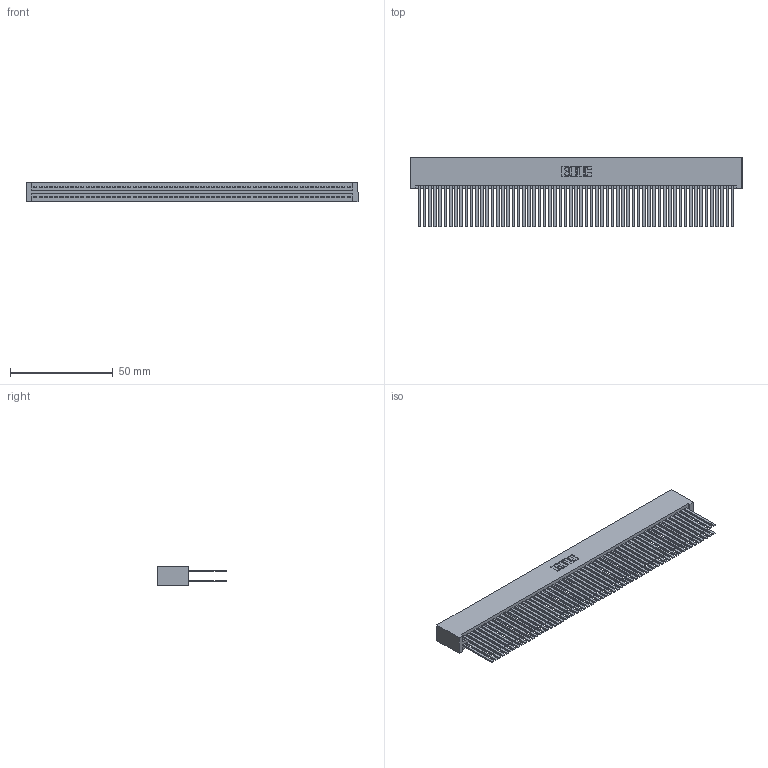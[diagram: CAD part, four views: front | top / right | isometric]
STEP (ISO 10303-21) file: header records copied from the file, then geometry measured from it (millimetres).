
FILE_DESCRIPTION (( 'STEP AP203' ), '1' );
FILE_NAME ('395-122-544-201.STEP', '2018-12-03T19:09:06', ( '' ), ( '' ), 'SwSTEP 2.0', 'SolidWorks 2016', '' );
FILE_SCHEMA (( 'CONFIG_CONTROL_DESIGN' ));
Length unit declared in the file: inch
Products named in the file (3): 345-292-001_345-293-144; 345 Part_No Mounting Lugs; 395-122-544-201
Assembly tree (123 placements, depth 2):
  395-122-544-201
    345 Part_No Mounting Lugs
    345-292-001_345-293-144  x122
Bounding box: 161.54 x 33.96 x 9.4 mm (x, y, z)
Volume: 18195 mm3; surface area: 32579.1 mm2
Topology: 123 solids, 123 shells, 5486 faces, 16299 edges, 10702 vertices
Faces by surface type: plane 3614, cylinder 1872
Entity records: 44843 total; most frequent: CARTESIAN_POINT 7496, ORIENTED_EDGE 7430, DIRECTION 6579, EDGE_CURVE 3715, LINE 3351, VECTOR 3351, VERTEX_POINT 2474, AXIS2_PLACEMENT_3D 1614
